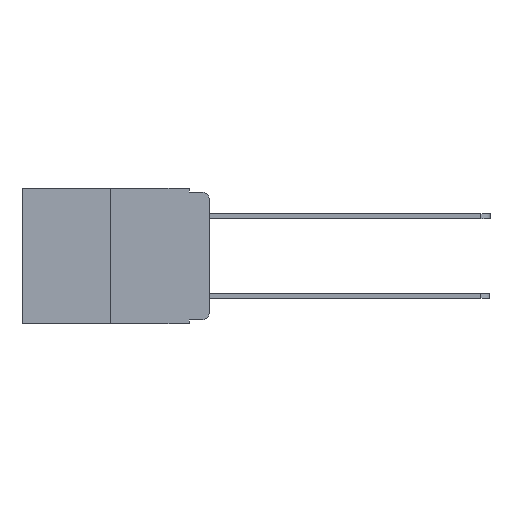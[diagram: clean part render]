
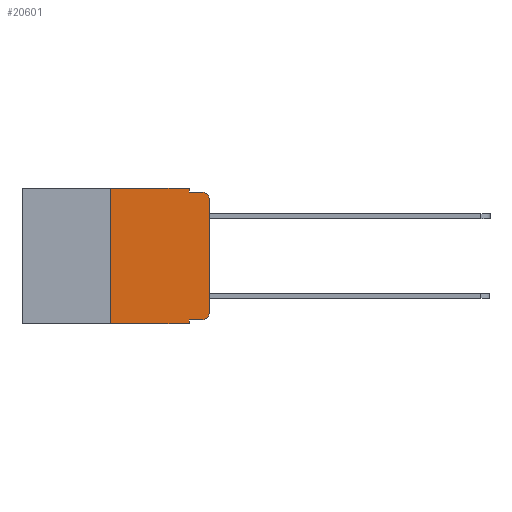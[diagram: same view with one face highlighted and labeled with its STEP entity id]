
A CAD part, left-side view. The second image highlights one B-rep face of the part: STEP entity #20601.
In plain terms, the highlighted planar face has unit normal (-1, 0, 0).
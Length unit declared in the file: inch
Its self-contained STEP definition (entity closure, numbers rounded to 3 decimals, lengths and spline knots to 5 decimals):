
#186 = DIRECTION ( 'NONE',  ( 0., -1., 0. ) ) ;
#425 = CARTESIAN_POINT ( 'NONE',  ( 0., 0.02, -0.01 ) ) ;
#624 = VECTOR ( 'NONE', #16985, 39.37008 ) ;
#1703 = CARTESIAN_POINT ( 'NONE',  ( 0., 0.051, -0.01 ) ) ;
#1774 = CARTESIAN_POINT ( 'NONE',  ( 0., 0.25, -0.343 ) ) ;
#1819 = CARTESIAN_POINT ( 'NONE',  ( 0., 0.051, -0.343 ) ) ;
#2198 = EDGE_CURVE ( 'NONE', #2323, #2392, #7220, .T. ) ;
#2243 = CARTESIAN_POINT ( 'NONE',  ( 0., 0.25, 0. ) ) ;
#2323 = VERTEX_POINT ( 'NONE', #16219 ) ;
#2392 = VERTEX_POINT ( 'NONE', #425 ) ;
#2636 = CARTESIAN_POINT ( 'NONE',  ( 0., 0.02, -0.333 ) ) ;
#2652 = CARTESIAN_POINT ( 'NONE',  ( 0., 0.051, -0.333 ) ) ;
#2808 = CARTESIAN_POINT ( 'NONE',  ( 0., 0.02, -0.313 ) ) ;
#3236 = PLANE ( 'NONE',  #17975 ) ;
#3343 = LINE ( 'NONE', #8031, #12298 ) ;
#3452 = VERTEX_POINT ( 'NONE', #5731 ) ;
#3528 = DIRECTION ( 'NONE',  ( 0., -1., 0. ) ) ;
#3726 = VERTEX_POINT ( 'NONE', #2636 ) ;
#4451 = AXIS2_PLACEMENT_3D ( 'NONE', #10555, #22607, #12317 ) ;
#4482 = DIRECTION ( 'NONE',  ( 0., -1., 0. ) ) ;
#4534 = DIRECTION ( 'NONE',  ( 0., 0., 1. ) ) ;
#4630 = DIRECTION ( 'NONE',  ( 0., 0., -1. ) ) ;
#5176 = CIRCLE ( 'NONE', #4451, 0.02 ) ;
#5540 = VERTEX_POINT ( 'NONE', #2243 ) ;
#5698 = EDGE_CURVE ( 'NONE', #7947, #5540, #14337, .T. ) ;
#5731 = CARTESIAN_POINT ( 'NONE',  ( 0., 0.051, 0. ) ) ;
#6182 = EDGE_CURVE ( 'NONE', #5540, #3452, #8559, .T. ) ;
#6546 = ORIENTED_EDGE ( 'NONE', *, *, #2198, .F. ) ;
#6660 = ORIENTED_EDGE ( 'NONE', *, *, #5698, .F. ) ;
#6934 = EDGE_LOOP ( 'NONE', ( #9615, #15811, #6546, #10136, #10435, #6660, #22147, #22416, #13145, #14519 ) ) ;
#7220 = LINE ( 'NONE', #1703, #19540 ) ;
#7947 = VERTEX_POINT ( 'NONE', #1774 ) ;
#8031 = CARTESIAN_POINT ( 'NONE',  ( 0., 0.051, 0. ) ) ;
#8444 = VECTOR ( 'NONE', #4482, 39.37008 ) ;
#8559 = LINE ( 'NONE', #14457, #21867 ) ;
#8610 = VERTEX_POINT ( 'NONE', #1819 ) ;
#9608 = EDGE_CURVE ( 'NONE', #22477, #3726, #12899, .T. ) ;
#9615 = ORIENTED_EDGE ( 'NONE', *, *, #14280, .T. ) ;
#9924 = AXIS2_PLACEMENT_3D ( 'NONE', #2808, #15248, #4630 ) ;
#10136 = ORIENTED_EDGE ( 'NONE', *, *, #10937, .F. ) ;
#10198 = VECTOR ( 'NONE', #19172, 39.37008 ) ;
#10435 = ORIENTED_EDGE ( 'NONE', *, *, #6182, .F. ) ;
#10475 = CARTESIAN_POINT ( 'NONE',  ( 0., 0.473, 0. ) ) ;
#10555 = CARTESIAN_POINT ( 'NONE',  ( 0., 0.02, -0.03 ) ) ;
#10667 = CARTESIAN_POINT ( 'NONE',  ( 0., 0., -0.03 ) ) ;
#10937 = EDGE_CURVE ( 'NONE', #3452, #2323, #3343, .T. ) ;
#11806 = FACE_OUTER_BOUND ( 'NONE', #6934, .T. ) ;
#12233 = DIRECTION ( 'NONE',  ( 0., 0., -1. ) ) ;
#12298 = VECTOR ( 'NONE', #22012, 39.37008 ) ;
#12317 = DIRECTION ( 'NONE',  ( 0., 0., -1. ) ) ;
#12538 = CARTESIAN_POINT ( 'NONE',  ( 0., 0.051, -0.333 ) ) ;
#12899 = LINE ( 'NONE', #2652, #8444 ) ;
#12965 = CARTESIAN_POINT ( 'NONE',  ( 0., 0.473, -0.343 ) ) ;
#13145 = ORIENTED_EDGE ( 'NONE', *, *, #9608, .T. ) ;
#13496 = CARTESIAN_POINT ( 'NONE',  ( 0., 0.051, 0. ) ) ;
#13674 = EDGE_CURVE ( 'NONE', #21330, #2392, #5176, .T. ) ;
#13815 = VECTOR ( 'NONE', #4534, 39.37008 ) ;
#13944 = CARTESIAN_POINT ( 'NONE',  ( 0., 0., 0. ) ) ;
#14073 = VERTEX_POINT ( 'NONE', #16917 ) ;
#14280 = EDGE_CURVE ( 'NONE', #14073, #21330, #14837, .T. ) ;
#14337 = LINE ( 'NONE', #18608, #13815 ) ;
#14457 = CARTESIAN_POINT ( 'NONE',  ( 0., 0.473, 0. ) ) ;
#14519 = ORIENTED_EDGE ( 'NONE', *, *, #17345, .T. ) ;
#14709 = DIRECTION ( 'NONE',  ( 0., -1., 0. ) ) ;
#14837 = LINE ( 'NONE', #13944, #10198 ) ;
#15248 = DIRECTION ( 'NONE',  ( -1., 0., 0. ) ) ;
#15811 = ORIENTED_EDGE ( 'NONE', *, *, #13674, .T. ) ;
#16219 = CARTESIAN_POINT ( 'NONE',  ( 0., 0.051, -0.01 ) ) ;
#16917 = CARTESIAN_POINT ( 'NONE',  ( 0., 0., -0.313 ) ) ;
#16985 = DIRECTION ( 'NONE',  ( 0., 0., -1. ) ) ;
#17191 = EDGE_CURVE ( 'NONE', #7947, #8610, #17371, .T. ) ;
#17345 = EDGE_CURVE ( 'NONE', #3726, #14073, #22701, .T. ) ;
#17371 = LINE ( 'NONE', #12965, #21424 ) ;
#17975 = AXIS2_PLACEMENT_3D ( 'NONE', #10475, #22534, #12233 ) ;
#18608 = CARTESIAN_POINT ( 'NONE',  ( 0., 0.25, 0. ) ) ;
#18908 = LINE ( 'NONE', #13496, #624 ) ;
#19172 = DIRECTION ( 'NONE',  ( 0., 0., 1. ) ) ;
#19371 = EDGE_CURVE ( 'NONE', #22477, #8610, #18908, .T. ) ;
#19540 = VECTOR ( 'NONE', #3528, 39.37008 ) ;
#20601 = ADVANCED_FACE ( 'NONE', ( #11806 ), #3236, .F. ) ;
#21330 = VERTEX_POINT ( 'NONE', #10667 ) ;
#21424 = VECTOR ( 'NONE', #14709, 39.37008 ) ;
#21867 = VECTOR ( 'NONE', #186, 39.37008 ) ;
#22012 = DIRECTION ( 'NONE',  ( 0., 0., -1. ) ) ;
#22147 = ORIENTED_EDGE ( 'NONE', *, *, #17191, .T. ) ;
#22416 = ORIENTED_EDGE ( 'NONE', *, *, #19371, .F. ) ;
#22477 = VERTEX_POINT ( 'NONE', #12538 ) ;
#22534 = DIRECTION ( 'NONE',  ( 1., 0., 0. ) ) ;
#22607 = DIRECTION ( 'NONE',  ( -1., 0., 0. ) ) ;
#22701 = CIRCLE ( 'NONE', #9924, 0.02 ) ;
